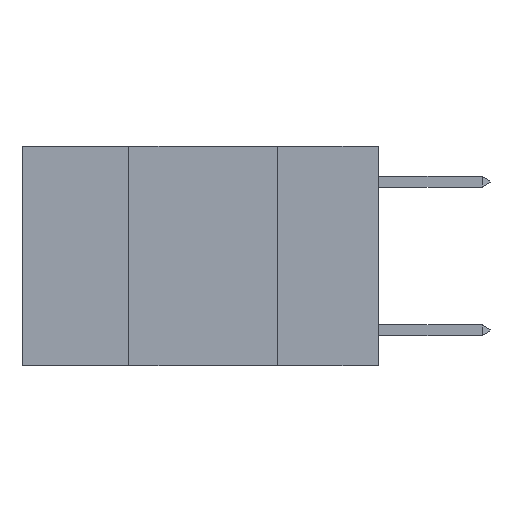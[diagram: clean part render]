
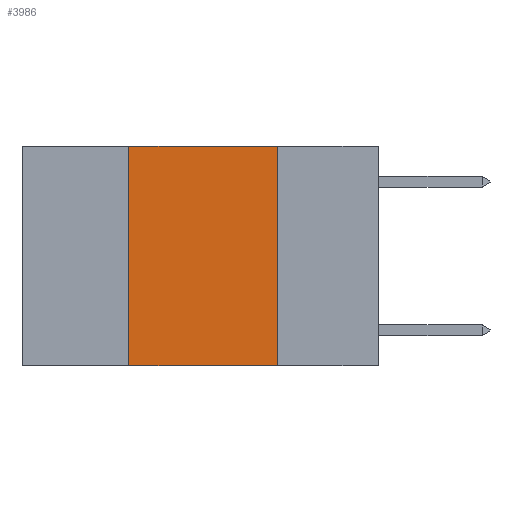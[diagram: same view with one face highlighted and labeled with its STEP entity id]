
A CAD part, left-side view. The second image highlights one B-rep face of the part: STEP entity #3986.
In plain terms, the highlighted planar face has unit normal (-1, 0, 0).
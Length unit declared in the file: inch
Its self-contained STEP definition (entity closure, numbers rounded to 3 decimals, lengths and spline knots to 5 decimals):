
#287 = PLANE ( 'NONE',  #8653 ) ;
#426 = LINE ( 'NONE', #5478, #8883 ) ;
#619 = VECTOR ( 'NONE', #5518, 39.37008 ) ;
#973 = VERTEX_POINT ( 'NONE', #3359 ) ;
#1024 = CARTESIAN_POINT ( 'NONE',  ( 0., 0.42, -0.37 ) ) ;
#1245 = VECTOR ( 'NONE', #10437, 39.37008 ) ;
#1504 = VECTOR ( 'NONE', #4800, 39.37008 ) ;
#1550 = LINE ( 'NONE', #5505, #1504 ) ;
#1789 = ORIENTED_EDGE ( 'NONE', *, *, #6123, .F. ) ;
#1862 = CARTESIAN_POINT ( 'NONE',  ( 0., 0.6, 0. ) ) ;
#2984 = CARTESIAN_POINT ( 'NONE',  ( 0., 0.17, 0. ) ) ;
#3204 = VERTEX_POINT ( 'NONE', #7712 ) ;
#3359 = CARTESIAN_POINT ( 'NONE',  ( 0., 0.17, -0.37 ) ) ;
#3635 = VERTEX_POINT ( 'NONE', #2984 ) ;
#3892 = ORIENTED_EDGE ( 'NONE', *, *, #4432, .T. ) ;
#3986 = ADVANCED_FACE ( 'NONE', ( #5920 ), #287, .F. ) ;
#4007 = ORIENTED_EDGE ( 'NONE', *, *, #10427, .F. ) ;
#4063 = DIRECTION ( 'NONE',  ( 0., 0., -1. ) ) ;
#4432 = EDGE_CURVE ( 'NONE', #4553, #973, #6329, .T. ) ;
#4553 = VERTEX_POINT ( 'NONE', #1024 ) ;
#4599 = LINE ( 'NONE', #7031, #1245 ) ;
#4717 = DIRECTION ( 'NONE',  ( 0., 0., 1. ) ) ;
#4800 = DIRECTION ( 'NONE',  ( 0., 0., -1. ) ) ;
#5478 = CARTESIAN_POINT ( 'NONE',  ( 0., 0.42, 0. ) ) ;
#5505 = CARTESIAN_POINT ( 'NONE',  ( 0., 0.17, 0. ) ) ;
#5518 = DIRECTION ( 'NONE',  ( 0., -1., 0. ) ) ;
#5920 = FACE_OUTER_BOUND ( 'NONE', #6036, .T. ) ;
#6036 = EDGE_LOOP ( 'NONE', ( #1789, #4007, #10125, #3892 ) ) ;
#6123 = EDGE_CURVE ( 'NONE', #3635, #973, #1550, .T. ) ;
#6329 = LINE ( 'NONE', #7875, #619 ) ;
#7031 = CARTESIAN_POINT ( 'NONE',  ( 0., 0.6, 0. ) ) ;
#7280 = EDGE_CURVE ( 'NONE', #4553, #3204, #426, .T. ) ;
#7712 = CARTESIAN_POINT ( 'NONE',  ( 0., 0.42, 0. ) ) ;
#7875 = CARTESIAN_POINT ( 'NONE',  ( 0., 0.6, -0.37 ) ) ;
#8653 = AXIS2_PLACEMENT_3D ( 'NONE', #1862, #8921, #4063 ) ;
#8883 = VECTOR ( 'NONE', #4717, 39.37008 ) ;
#8921 = DIRECTION ( 'NONE',  ( 1., 0., 0. ) ) ;
#10125 = ORIENTED_EDGE ( 'NONE', *, *, #7280, .F. ) ;
#10427 = EDGE_CURVE ( 'NONE', #3204, #3635, #4599, .T. ) ;
#10437 = DIRECTION ( 'NONE',  ( 0., -1., 0. ) ) ;
